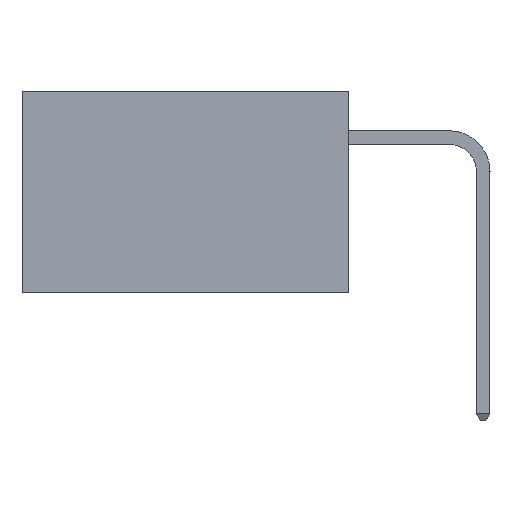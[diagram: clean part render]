
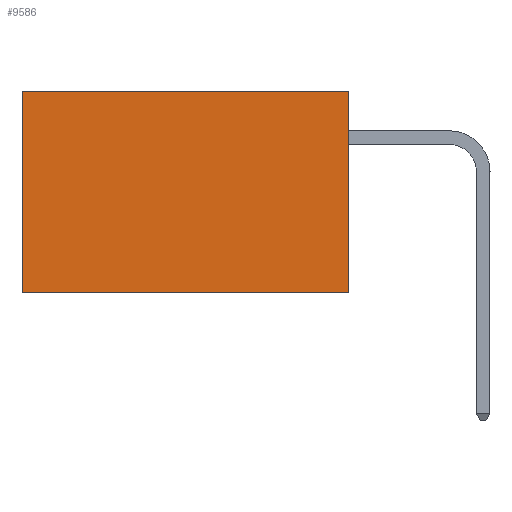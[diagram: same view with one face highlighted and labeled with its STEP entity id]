
A CAD part, left-side view. The second image highlights one B-rep face of the part: STEP entity #9586.
In plain terms, the highlighted planar face has unit normal (-1, 0, 0).
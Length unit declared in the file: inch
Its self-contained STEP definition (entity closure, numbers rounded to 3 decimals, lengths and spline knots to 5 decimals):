
#1005 = CARTESIAN_POINT ( 'NONE',  ( 0.2875, 0.6, 0. ) ) ;
#3823 = VERTEX_POINT ( 'NONE', #15326 ) ;
#4174 = ORIENTED_EDGE ( 'NONE', *, *, #37858, .F. ) ;
#9276 = EDGE_LOOP ( 'NONE', ( #39686, #9761, #4174, #38977 ) ) ;
#9586 = ADVANCED_FACE ( 'NONE', ( #34746 ), #39312, .F. ) ;
#9761 = ORIENTED_EDGE ( 'NONE', *, *, #14112, .F. ) ;
#10108 = VECTOR ( 'NONE', #30289, 39.37008 ) ;
#10582 = LINE ( 'NONE', #17087, #10108 ) ;
#11868 = VECTOR ( 'NONE', #12304, 39.37008 ) ;
#12170 = CARTESIAN_POINT ( 'NONE',  ( 0.2875, 0., 0. ) ) ;
#12304 = DIRECTION ( 'NONE',  ( 0., 1., 0. ) ) ;
#14112 = EDGE_CURVE ( 'NONE', #30200, #3823, #29252, .T. ) ;
#15326 = CARTESIAN_POINT ( 'NONE',  ( 0.2875, 0.6, -0.37 ) ) ;
#17087 = CARTESIAN_POINT ( 'NONE',  ( 0.2875, 0., 0. ) ) ;
#17867 = DIRECTION ( 'NONE',  ( 1., 0., 0. ) ) ;
#20426 = EDGE_CURVE ( 'NONE', #40213, #3823, #30102, .T. ) ;
#22380 = EDGE_CURVE ( 'NONE', #31120, #40213, #10582, .T. ) ;
#22421 = CARTESIAN_POINT ( 'NONE',  ( 0.2875, 0., 0. ) ) ;
#22706 = CARTESIAN_POINT ( 'NONE',  ( 0.2875, 0., -0.37 ) ) ;
#23818 = LINE ( 'NONE', #22421, #37796 ) ;
#24844 = CARTESIAN_POINT ( 'NONE',  ( 0.2875, 0., -0.37 ) ) ;
#29252 = LINE ( 'NONE', #24844, #11868 ) ;
#30102 = LINE ( 'NONE', #35114, #33585 ) ;
#30200 = VERTEX_POINT ( 'NONE', #22706 ) ;
#30289 = DIRECTION ( 'NONE',  ( 0., 1., 0. ) ) ;
#30535 = CARTESIAN_POINT ( 'NONE',  ( 0.2875, 0., 0. ) ) ;
#31120 = VERTEX_POINT ( 'NONE', #12170 ) ;
#31984 = AXIS2_PLACEMENT_3D ( 'NONE', #30535, #17867, #36804 ) ;
#33585 = VECTOR ( 'NONE', #35248, 39.37008 ) ;
#34709 = DIRECTION ( 'NONE',  ( 0., 0., -1. ) ) ;
#34746 = FACE_OUTER_BOUND ( 'NONE', #9276, .T. ) ;
#35114 = CARTESIAN_POINT ( 'NONE',  ( 0.2875, 0.6, 0. ) ) ;
#35248 = DIRECTION ( 'NONE',  ( 0., 0., -1. ) ) ;
#36804 = DIRECTION ( 'NONE',  ( 0., 0., -1. ) ) ;
#37796 = VECTOR ( 'NONE', #34709, 39.37008 ) ;
#37858 = EDGE_CURVE ( 'NONE', #31120, #30200, #23818, .T. ) ;
#38977 = ORIENTED_EDGE ( 'NONE', *, *, #22380, .T. ) ;
#39312 = PLANE ( 'NONE',  #31984 ) ;
#39686 = ORIENTED_EDGE ( 'NONE', *, *, #20426, .T. ) ;
#40213 = VERTEX_POINT ( 'NONE', #1005 ) ;
